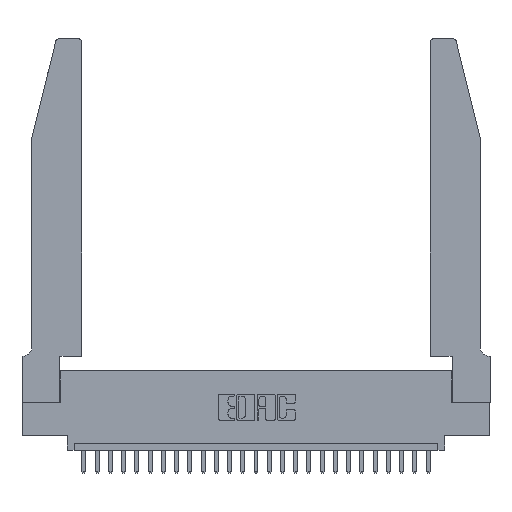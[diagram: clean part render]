
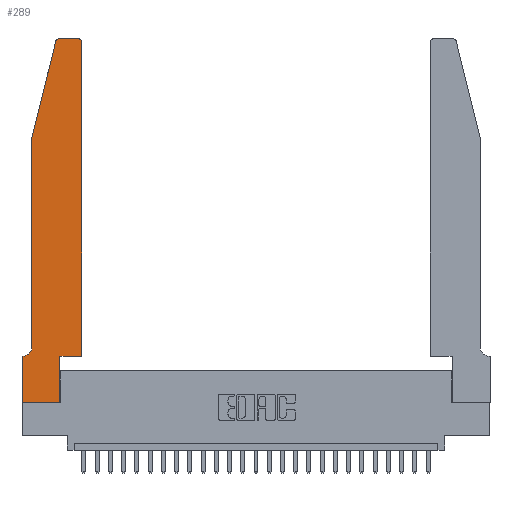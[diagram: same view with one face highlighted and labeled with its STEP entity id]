
A CAD part, top view. The second image highlights one B-rep face of the part: STEP entity #289.
In plain terms, the highlighted planar face has unit normal (0, 0, 1).
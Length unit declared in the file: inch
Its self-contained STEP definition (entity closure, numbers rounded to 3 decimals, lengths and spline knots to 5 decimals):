
#80 = LINE ( 'NONE', #21202, #15548 ) ;
#150 = VECTOR ( 'NONE', #1090, 39.37008 ) ;
#183 = VERTEX_POINT ( 'NONE', #14788 ) ;
#251 = CARTESIAN_POINT ( 'NONE',  ( 0.4505, 0.35, 0.37 ) ) ;
#289 = ADVANCED_FACE ( 'NONE', ( #12936 ), #13726, .T. ) ;
#618 = EDGE_CURVE ( 'NONE', #12095, #15433, #80, .T. ) ;
#662 = ORIENTED_EDGE ( 'NONE', *, *, #15666, .T. ) ;
#861 = LINE ( 'NONE', #17011, #4503 ) ;
#1073 = DIRECTION ( 'NONE',  ( 0., 0., 1. ) ) ;
#1090 = DIRECTION ( 'NONE',  ( 0., 1., 0. ) ) ;
#1300 = VECTOR ( 'NONE', #2524, 39.37008 ) ;
#1319 = ORIENTED_EDGE ( 'NONE', *, *, #6160, .T. ) ;
#1455 = ORIENTED_EDGE ( 'NONE', *, *, #22760, .T. ) ;
#1658 = DIRECTION ( 'NONE',  ( 0., 0., 1. ) ) ;
#1756 = ORIENTED_EDGE ( 'NONE', *, *, #2145, .T. ) ;
#2145 = EDGE_CURVE ( 'NONE', #6424, #4406, #2988, .T. ) ;
#2503 = DIRECTION ( 'NONE',  ( 1., 0., 0. ) ) ;
#2524 = DIRECTION ( 'NONE',  ( -1., 0., 0. ) ) ;
#2667 = AXIS2_PLACEMENT_3D ( 'NONE', #18255, #13752, #24433 ) ;
#2707 = DIRECTION ( 'NONE',  ( 1., 0., 0. ) ) ;
#2988 = CIRCLE ( 'NONE', #2667, 0.07 ) ;
#3865 = CARTESIAN_POINT ( 'NONE',  ( 0.0755, 2., 0.37 ) ) ;
#4406 = VERTEX_POINT ( 'NONE', #19811 ) ;
#4426 = DIRECTION ( 'NONE',  ( -0.239, -0.971, 0. ) ) ;
#4503 = VECTOR ( 'NONE', #4426, 39.37008 ) ;
#4860 = CARTESIAN_POINT ( 'NONE',  ( 0., 0.35, 0.37 ) ) ;
#4922 = AXIS2_PLACEMENT_3D ( 'NONE', #5545, #7190, #22125 ) ;
#4951 = CARTESIAN_POINT ( 'NONE',  ( 0.2865, 0.35, 0.37 ) ) ;
#5126 = DIRECTION ( 'NONE',  ( 0., -1., 0. ) ) ;
#5545 = CARTESIAN_POINT ( 'NONE',  ( 0., 0.35, 0.37 ) ) ;
#5574 = ORIENTED_EDGE ( 'NONE', *, *, #13035, .T. ) ;
#6160 = EDGE_CURVE ( 'NONE', #15433, #183, #18994, .T. ) ;
#6424 = VERTEX_POINT ( 'NONE', #21921 ) ;
#6573 = EDGE_CURVE ( 'NONE', #26957, #23141, #861, .T. ) ;
#6686 = EDGE_CURVE ( 'NONE', #24276, #19834, #19280, .T. ) ;
#6767 = DIRECTION ( 'NONE',  ( -1., 0., 0. ) ) ;
#6955 = LINE ( 'NONE', #15613, #19126 ) ;
#7033 = CARTESIAN_POINT ( 'NONE',  ( 0.0755, 0.35, 0.37 ) ) ;
#7190 = DIRECTION ( 'NONE',  ( 0., 0., 1. ) ) ;
#7244 = ORIENTED_EDGE ( 'NONE', *, *, #25732, .T. ) ;
#7424 = CIRCLE ( 'NONE', #11157, 0.03 ) ;
#7999 = CARTESIAN_POINT ( 'NONE',  ( 0.4205, 2.72, 0.37 ) ) ;
#8852 = VECTOR ( 'NONE', #6767, 39.37008 ) ;
#9133 = EDGE_CURVE ( 'NONE', #23141, #6424, #9281, .T. ) ;
#9281 = LINE ( 'NONE', #13172, #19859 ) ;
#11027 = CARTESIAN_POINT ( 'NONE',  ( 0.4505, 0.35, 0.37 ) ) ;
#11094 = EDGE_LOOP ( 'NONE', ( #7244, #12044, #21166, #24777, #1756, #22658, #1455, #24258, #5574, #11887, #1319, #662 ) ) ;
#11157 = AXIS2_PLACEMENT_3D ( 'NONE', #22061, #1073, #11353 ) ;
#11353 = DIRECTION ( 'NONE',  ( 1., 0., 0. ) ) ;
#11768 = VECTOR ( 'NONE', #15159, 39.37008 ) ;
#11855 = CIRCLE ( 'NONE', #19932, 0.03 ) ;
#11887 = ORIENTED_EDGE ( 'NONE', *, *, #618, .T. ) ;
#12044 = ORIENTED_EDGE ( 'NONE', *, *, #19971, .T. ) ;
#12095 = VERTEX_POINT ( 'NONE', #15288 ) ;
#12208 = LINE ( 'NONE', #7033, #8852 ) ;
#12936 = FACE_OUTER_BOUND ( 'NONE', #11094, .T. ) ;
#13035 = EDGE_CURVE ( 'NONE', #19834, #12095, #20267, .T. ) ;
#13172 = CARTESIAN_POINT ( 'NONE',  ( 0.0755, 2., 0.37 ) ) ;
#13726 = PLANE ( 'NONE',  #4922 ) ;
#13752 = DIRECTION ( 'NONE',  ( 0., 0., -1. ) ) ;
#14788 = CARTESIAN_POINT ( 'NONE',  ( 0.4505, 2.72, 0.37 ) ) ;
#15159 = DIRECTION ( 'NONE',  ( 0., 1., 0. ) ) ;
#15288 = CARTESIAN_POINT ( 'NONE',  ( 0.2865, 0.35, 0.37 ) ) ;
#15297 = CARTESIAN_POINT ( 'NONE',  ( 0.4205, 2.75, 0.37 ) ) ;
#15358 = CARTESIAN_POINT ( 'NONE',  ( 0.2605, 2.75, 0.37 ) ) ;
#15433 = VERTEX_POINT ( 'NONE', #251 ) ;
#15548 = VECTOR ( 'NONE', #2503, 39.37008 ) ;
#15613 = CARTESIAN_POINT ( 'NONE',  ( 0., 0., 0.37 ) ) ;
#15666 = EDGE_CURVE ( 'NONE', #183, #17220, #11855, .T. ) ;
#16743 = CARTESIAN_POINT ( 'NONE',  ( 0.2865, 0., 0.37 ) ) ;
#17011 = CARTESIAN_POINT ( 'NONE',  ( 0.0755, 2., 0.37 ) ) ;
#17220 = VERTEX_POINT ( 'NONE', #15297 ) ;
#18255 = CARTESIAN_POINT ( 'NONE',  ( 0.0055, 0.42, 0.37 ) ) ;
#18396 = CARTESIAN_POINT ( 'NONE',  ( 0., 0., 0.37 ) ) ;
#18994 = LINE ( 'NONE', #11027, #11768 ) ;
#19126 = VECTOR ( 'NONE', #5126, 39.37008 ) ;
#19280 = LINE ( 'NONE', #19822, #21942 ) ;
#19811 = CARTESIAN_POINT ( 'NONE',  ( 0.0055, 0.35, 0.37 ) ) ;
#19822 = CARTESIAN_POINT ( 'NONE',  ( 0., 0., 0.37 ) ) ;
#19834 = VERTEX_POINT ( 'NONE', #16743 ) ;
#19859 = VECTOR ( 'NONE', #23425, 39.37008 ) ;
#19932 = AXIS2_PLACEMENT_3D ( 'NONE', #7999, #1658, #20625 ) ;
#19971 = EDGE_CURVE ( 'NONE', #26499, #26957, #7424, .T. ) ;
#20267 = LINE ( 'NONE', #4951, #150 ) ;
#20454 = CARTESIAN_POINT ( 'NONE',  ( 0.284, 2.75, 0.37 ) ) ;
#20625 = DIRECTION ( 'NONE',  ( 1., 0., 0. ) ) ;
#20753 = VERTEX_POINT ( 'NONE', #4860 ) ;
#21166 = ORIENTED_EDGE ( 'NONE', *, *, #6573, .T. ) ;
#21202 = CARTESIAN_POINT ( 'NONE',  ( 0.4505, 0.35, 0.37 ) ) ;
#21706 = LINE ( 'NONE', #15358, #1300 ) ;
#21894 = CARTESIAN_POINT ( 'NONE',  ( 0.25487, 2.72718, 0.37 ) ) ;
#21921 = CARTESIAN_POINT ( 'NONE',  ( 0.0755, 0.42, 0.37 ) ) ;
#21942 = VECTOR ( 'NONE', #2707, 39.37008 ) ;
#22061 = CARTESIAN_POINT ( 'NONE',  ( 0.284, 2.72, 0.37 ) ) ;
#22125 = DIRECTION ( 'NONE',  ( 1., 0., 0. ) ) ;
#22658 = ORIENTED_EDGE ( 'NONE', *, *, #23308, .T. ) ;
#22760 = EDGE_CURVE ( 'NONE', #20753, #24276, #6955, .T. ) ;
#23141 = VERTEX_POINT ( 'NONE', #3865 ) ;
#23308 = EDGE_CURVE ( 'NONE', #4406, #20753, #12208, .T. ) ;
#23425 = DIRECTION ( 'NONE',  ( 0., -1., 0. ) ) ;
#24258 = ORIENTED_EDGE ( 'NONE', *, *, #6686, .T. ) ;
#24276 = VERTEX_POINT ( 'NONE', #18396 ) ;
#24433 = DIRECTION ( 'NONE',  ( -1., 0., 0. ) ) ;
#24777 = ORIENTED_EDGE ( 'NONE', *, *, #9133, .T. ) ;
#25732 = EDGE_CURVE ( 'NONE', #17220, #26499, #21706, .T. ) ;
#26499 = VERTEX_POINT ( 'NONE', #20454 ) ;
#26957 = VERTEX_POINT ( 'NONE', #21894 ) ;
